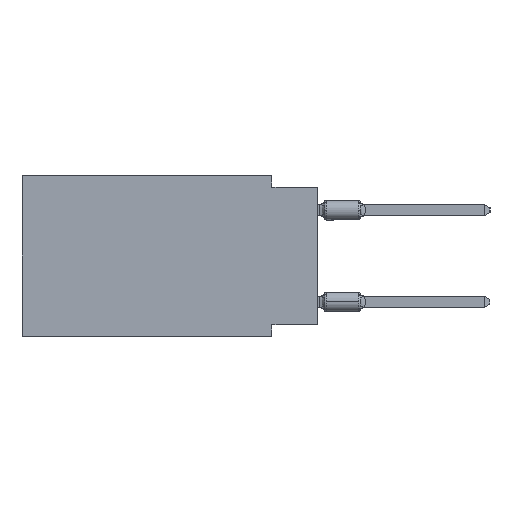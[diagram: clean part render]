
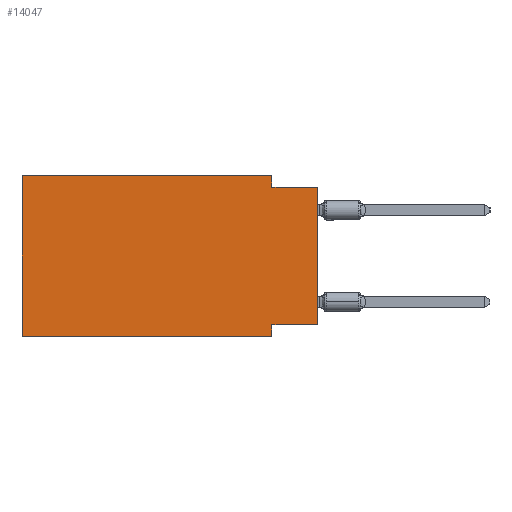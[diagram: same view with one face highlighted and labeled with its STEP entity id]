
A CAD part, left-side view. The second image highlights one B-rep face of the part: STEP entity #14047.
In plain terms, the highlighted planar face has unit normal (-1, 0, 0).
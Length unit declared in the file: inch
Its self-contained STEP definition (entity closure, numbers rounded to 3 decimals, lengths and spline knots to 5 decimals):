
#647 = CARTESIAN_POINT ( 'NONE',  ( 0., 0.1, 0. ) ) ;
#3004 = ORIENTED_EDGE ( 'NONE', *, *, #14523, .F. ) ;
#4061 = DIRECTION ( 'NONE',  ( 0., -1., 0. ) ) ;
#5492 = CARTESIAN_POINT ( 'NONE',  ( 0., 0., -0.325 ) ) ;
#6056 = CARTESIAN_POINT ( 'NONE',  ( 0., 0., -0.325 ) ) ;
#7916 = ORIENTED_EDGE ( 'NONE', *, *, #61150, .F. ) ;
#8618 = VERTEX_POINT ( 'NONE', #48631 ) ;
#10442 = DIRECTION ( 'NONE',  ( 1., 0., 0. ) ) ;
#13901 = VECTOR ( 'NONE', #62959, 39.37008 ) ;
#14047 = ADVANCED_FACE ( 'NONE', ( #31545 ), #63250, .F. ) ;
#14086 = CARTESIAN_POINT ( 'NONE',  ( 0., 0.645, 0. ) ) ;
#14523 = EDGE_CURVE ( 'NONE', #59449, #51325, #26435, .T. ) ;
#15890 = DIRECTION ( 'NONE',  ( 0., 0., -1. ) ) ;
#17130 = EDGE_CURVE ( 'NONE', #58039, #8618, #42855, .T. ) ;
#19286 = EDGE_CURVE ( 'NONE', #28977, #59449, #52820, .T. ) ;
#19470 = VECTOR ( 'NONE', #4061, 39.37008 ) ;
#20584 = VERTEX_POINT ( 'NONE', #63705 ) ;
#20761 = CARTESIAN_POINT ( 'NONE',  ( 0., 0.645, 0. ) ) ;
#20779 = ORIENTED_EDGE ( 'NONE', *, *, #17130, .F. ) ;
#20807 = AXIS2_PLACEMENT_3D ( 'NONE', #52329, #10442, #26106 ) ;
#21466 = DIRECTION ( 'NONE',  ( 0., 1., 0. ) ) ;
#23285 = LINE ( 'NONE', #14086, #49043 ) ;
#26106 = DIRECTION ( 'NONE',  ( 0., 0., -1. ) ) ;
#26435 = LINE ( 'NONE', #27096, #37163 ) ;
#27096 = CARTESIAN_POINT ( 'NONE',  ( 0., 0.1, -0.35 ) ) ;
#28977 = VERTEX_POINT ( 'NONE', #6056 ) ;
#29946 = CARTESIAN_POINT ( 'NONE',  ( 0., 0.645, -0.35 ) ) ;
#30118 = DIRECTION ( 'NONE',  ( 0., 0., 1. ) ) ;
#31545 = FACE_OUTER_BOUND ( 'NONE', #52970, .T. ) ;
#31759 = DIRECTION ( 'NONE',  ( 0., -1., 0. ) ) ;
#32893 = CARTESIAN_POINT ( 'NONE',  ( 0., 0.1, 0. ) ) ;
#36323 = EDGE_CURVE ( 'NONE', #52694, #51325, #45275, .T. ) ;
#36415 = DIRECTION ( 'NONE',  ( 0., -1., 0. ) ) ;
#37163 = VECTOR ( 'NONE', #15890, 39.37008 ) ;
#38421 = EDGE_CURVE ( 'NONE', #52694, #20584, #23285, .T. ) ;
#42855 = LINE ( 'NONE', #647, #13901 ) ;
#44824 = LINE ( 'NONE', #50597, #61133 ) ;
#44955 = CARTESIAN_POINT ( 'NONE',  ( 0., 0.645, -0.35 ) ) ;
#45275 = LINE ( 'NONE', #44955, #19470 ) ;
#45433 = ORIENTED_EDGE ( 'NONE', *, *, #19286, .F. ) ;
#47186 = ORIENTED_EDGE ( 'NONE', *, *, #38421, .F. ) ;
#47269 = ORIENTED_EDGE ( 'NONE', *, *, #54701, .T. ) ;
#48631 = CARTESIAN_POINT ( 'NONE',  ( 0., 0.1, -0.025 ) ) ;
#49043 = VECTOR ( 'NONE', #55644, 39.37008 ) ;
#50597 = CARTESIAN_POINT ( 'NONE',  ( 0., 0., 0. ) ) ;
#51325 = VERTEX_POINT ( 'NONE', #62604 ) ;
#52329 = CARTESIAN_POINT ( 'NONE',  ( 0., 0.645, 0. ) ) ;
#52535 = CARTESIAN_POINT ( 'NONE',  ( 0., 0., -0.025 ) ) ;
#52694 = VERTEX_POINT ( 'NONE', #29946 ) ;
#52820 = LINE ( 'NONE', #5492, #58737 ) ;
#52970 = EDGE_LOOP ( 'NONE', ( #47269, #64378, #20779, #7916, #47186, #57083, #3004, #45433 ) ) ;
#53099 = LINE ( 'NONE', #20761, #61541 ) ;
#53425 = CARTESIAN_POINT ( 'NONE',  ( 0., 0., -0.025 ) ) ;
#54063 = VERTEX_POINT ( 'NONE', #53425 ) ;
#54701 = EDGE_CURVE ( 'NONE', #28977, #54063, #44824, .T. ) ;
#55644 = DIRECTION ( 'NONE',  ( 0., 0., 1. ) ) ;
#57083 = ORIENTED_EDGE ( 'NONE', *, *, #36323, .T. ) ;
#58039 = VERTEX_POINT ( 'NONE', #32893 ) ;
#58381 = VECTOR ( 'NONE', #31759, 39.37008 ) ;
#58737 = VECTOR ( 'NONE', #21466, 39.37008 ) ;
#59449 = VERTEX_POINT ( 'NONE', #61571 ) ;
#61133 = VECTOR ( 'NONE', #30118, 39.37008 ) ;
#61150 = EDGE_CURVE ( 'NONE', #20584, #58039, #53099, .T. ) ;
#61541 = VECTOR ( 'NONE', #36415, 39.37008 ) ;
#61571 = CARTESIAN_POINT ( 'NONE',  ( 0., 0.1, -0.325 ) ) ;
#62030 = EDGE_CURVE ( 'NONE', #8618, #54063, #63765, .T. ) ;
#62604 = CARTESIAN_POINT ( 'NONE',  ( 0., 0.1, -0.35 ) ) ;
#62959 = DIRECTION ( 'NONE',  ( 0., 0., -1. ) ) ;
#63250 = PLANE ( 'NONE',  #20807 ) ;
#63705 = CARTESIAN_POINT ( 'NONE',  ( 0., 0.645, 0. ) ) ;
#63765 = LINE ( 'NONE', #52535, #58381 ) ;
#64378 = ORIENTED_EDGE ( 'NONE', *, *, #62030, .F. ) ;
